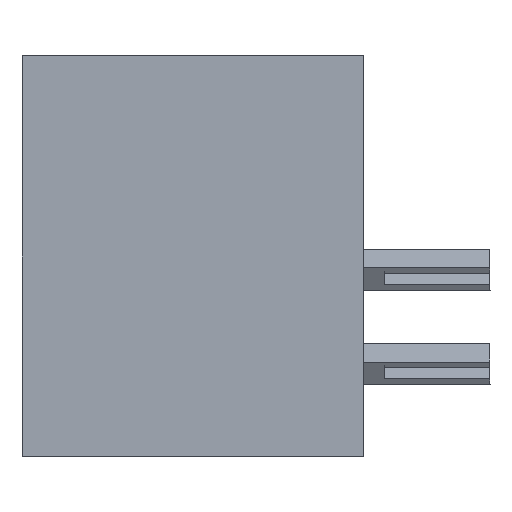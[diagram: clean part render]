
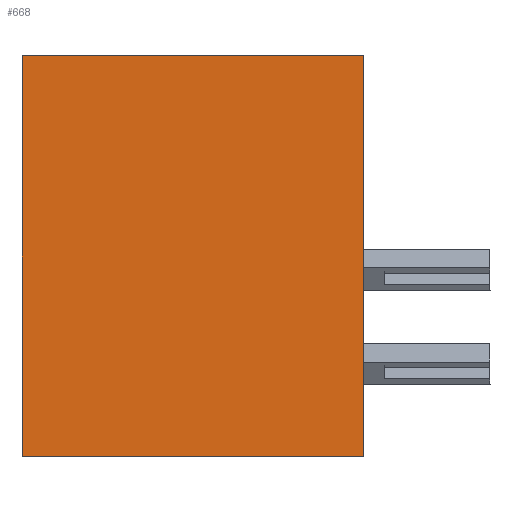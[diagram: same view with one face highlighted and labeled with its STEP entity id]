
A CAD part, left-side view. The second image highlights one B-rep face of the part: STEP entity #668.
In plain terms, the highlighted planar face has unit normal (-1, 0, 0).
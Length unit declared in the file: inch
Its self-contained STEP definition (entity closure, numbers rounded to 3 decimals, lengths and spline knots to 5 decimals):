
#19 = CARTESIAN_POINT ( 'NONE',  ( 0., 0.453, -0.531 ) ) ;
#302 = EDGE_LOOP ( 'NONE', ( #2013, #1991, #15031, #12832 ) ) ;
#412 = DIRECTION ( 'NONE',  ( 1., 0., 0. ) ) ;
#668 = ADVANCED_FACE ( 'NONE', ( #1021 ), #13942, .F. ) ;
#1021 = FACE_OUTER_BOUND ( 'NONE', #302, .T. ) ;
#1107 = LINE ( 'NONE', #16010, #2726 ) ;
#1610 = CARTESIAN_POINT ( 'NONE',  ( 0., 0.453, -0.531 ) ) ;
#1991 = ORIENTED_EDGE ( 'NONE', *, *, #5321, .F. ) ;
#2013 = ORIENTED_EDGE ( 'NONE', *, *, #15089, .T. ) ;
#2023 = DIRECTION ( 'NONE',  ( 0., 0., -1. ) ) ;
#2153 = EDGE_CURVE ( 'NONE', #4997, #13111, #6356, .T. ) ;
#2338 = CARTESIAN_POINT ( 'NONE',  ( 0., 0., 0. ) ) ;
#2726 = VECTOR ( 'NONE', #7079, 39.37008 ) ;
#3452 = VERTEX_POINT ( 'NONE', #6148 ) ;
#4457 = AXIS2_PLACEMENT_3D ( 'NONE', #18255, #412, #2023 ) ;
#4505 = CARTESIAN_POINT ( 'NONE',  ( 0., 0., 0. ) ) ;
#4997 = VERTEX_POINT ( 'NONE', #19 ) ;
#5114 = CARTESIAN_POINT ( 'NONE',  ( 0., 0.453, 0. ) ) ;
#5321 = EDGE_CURVE ( 'NONE', #13111, #11779, #1107, .T. ) ;
#5932 = CARTESIAN_POINT ( 'NONE',  ( 0., 0.453, 0. ) ) ;
#6148 = CARTESIAN_POINT ( 'NONE',  ( 0., 0., -0.531 ) ) ;
#6356 = LINE ( 'NONE', #5114, #14765 ) ;
#7079 = DIRECTION ( 'NONE',  ( 0., -1., 0. ) ) ;
#7517 = LINE ( 'NONE', #1610, #9136 ) ;
#8535 = DIRECTION ( 'NONE',  ( 0., -1., 0. ) ) ;
#9136 = VECTOR ( 'NONE', #8535, 39.37008 ) ;
#9188 = DIRECTION ( 'NONE',  ( 0., 0., 1. ) ) ;
#9664 = VECTOR ( 'NONE', #9188, 39.37008 ) ;
#11779 = VERTEX_POINT ( 'NONE', #2338 ) ;
#11976 = LINE ( 'NONE', #4505, #9664 ) ;
#12159 = EDGE_CURVE ( 'NONE', #4997, #3452, #7517, .T. ) ;
#12832 = ORIENTED_EDGE ( 'NONE', *, *, #12159, .T. ) ;
#13111 = VERTEX_POINT ( 'NONE', #5932 ) ;
#13942 = PLANE ( 'NONE',  #4457 ) ;
#14031 = DIRECTION ( 'NONE',  ( 0., 0., 1. ) ) ;
#14765 = VECTOR ( 'NONE', #14031, 39.37008 ) ;
#15031 = ORIENTED_EDGE ( 'NONE', *, *, #2153, .F. ) ;
#15089 = EDGE_CURVE ( 'NONE', #3452, #11779, #11976, .T. ) ;
#16010 = CARTESIAN_POINT ( 'NONE',  ( 0., 0.453, 0. ) ) ;
#18255 = CARTESIAN_POINT ( 'NONE',  ( 0., 0.453, 0. ) ) ;
